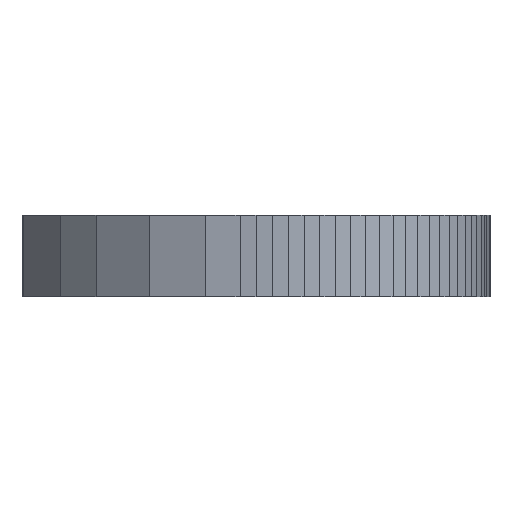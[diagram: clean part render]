
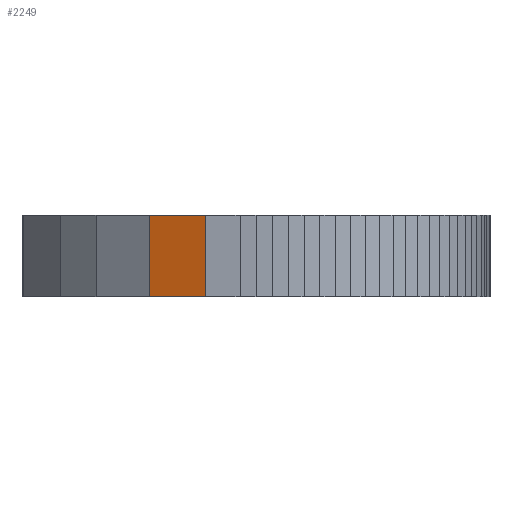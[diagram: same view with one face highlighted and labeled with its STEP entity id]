
A CAD part, left-side view. The second image highlights one B-rep face of the part: STEP entity #2249.
In plain terms, the highlighted planar face has unit normal (-0.933, 0.359, 0).
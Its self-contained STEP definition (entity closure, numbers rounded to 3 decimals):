
#2193=CARTESIAN_POINT('',(-34.199,4.912,0.0));
#2194=VERTEX_POINT('',#2193);
#2202=CARTESIAN_POINT('',(-34.199,4.912,11.0));
#2203=VERTEX_POINT('',#2202);
#2210=CARTESIAN_POINT('',(-34.199,4.912,0.0));
#2211=DIRECTION('',(0.0,0.0,1.0));
#2212=VECTOR('',#2211,11.0);
#2213=LINE('',#2210,#2212);
#2214=EDGE_CURVE('',#2194,#2203,#2213,.T.);
#2219=CARTESIAN_POINT('',(-31.291,12.47,0.0));
#2220=DIRECTION('',(-0.933,0.359,0.0));
#2221=DIRECTION('',(-0.359,-0.933,0.0));
#2222=AXIS2_PLACEMENT_3D('',#2219,#2220,#2221);
#2223=PLANE('',#2222);
#2224=CARTESIAN_POINT('',(-31.291,12.47,0.0));
#2225=VERTEX_POINT('',#2224);
#2226=CARTESIAN_POINT('',(-31.291,12.47,0.0));
#2227=DIRECTION('',(-0.359,-0.933,0.0));
#2228=VECTOR('',#2227,8.098);
#2229=LINE('',#2226,#2228);
#2230=EDGE_CURVE('',#2225,#2194,#2229,.T.);
#2231=ORIENTED_EDGE('',*,*,#2230,.T.);
#2232=ORIENTED_EDGE('',*,*,#2214,.T.);
#2233=CARTESIAN_POINT('',(-31.291,12.47,11.0));
#2234=VERTEX_POINT('',#2233);
#2235=CARTESIAN_POINT('',(-31.291,12.47,11.0));
#2236=DIRECTION('',(-0.359,-0.933,0.0));
#2237=VECTOR('',#2236,8.098);
#2238=LINE('',#2235,#2237);
#2239=EDGE_CURVE('',#2234,#2203,#2238,.T.);
#2240=ORIENTED_EDGE('',*,*,#2239,.F.);
#2241=CARTESIAN_POINT('',(-31.291,12.47,0.0));
#2242=DIRECTION('',(0.0,0.0,1.0));
#2243=VECTOR('',#2242,11.0);
#2244=LINE('',#2241,#2243);
#2245=EDGE_CURVE('',#2225,#2234,#2244,.T.);
#2246=ORIENTED_EDGE('',*,*,#2245,.F.);
#2247=EDGE_LOOP('',(#2231,#2232,#2240,#2246));
#2248=FACE_OUTER_BOUND('',#2247,.T.);
#2249=ADVANCED_FACE('',(#2248),#2223,.T.);
